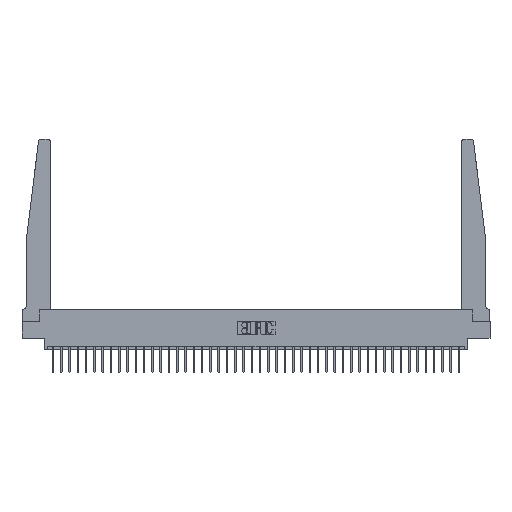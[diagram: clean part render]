
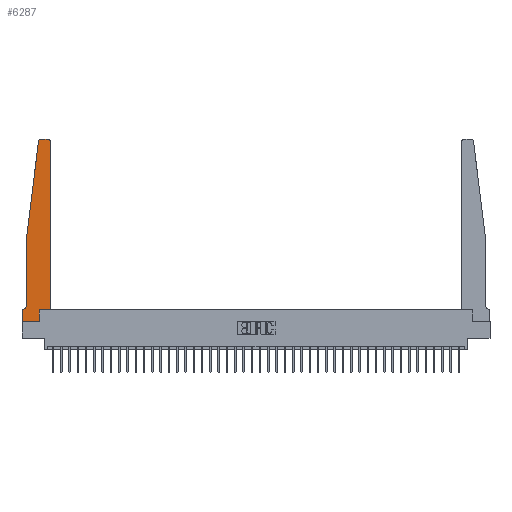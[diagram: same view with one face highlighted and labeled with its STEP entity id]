
A CAD part, top view. The second image highlights one B-rep face of the part: STEP entity #6287.
In plain terms, the highlighted planar face has unit normal (0, 0, 1).
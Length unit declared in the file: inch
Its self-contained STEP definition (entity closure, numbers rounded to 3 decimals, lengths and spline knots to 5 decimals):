
#651 = VECTOR ( 'NONE', #20652, 39.37008 ) ;
#763 = LINE ( 'NONE', #26192, #33918 ) ;
#776 = CARTESIAN_POINT ( 'NONE',  ( 0.27653, 2.75, 0.37 ) ) ;
#1004 = CARTESIAN_POINT ( 'NONE',  ( 0.065, 0.1875, 0.37 ) ) ;
#1012 = LINE ( 'NONE', #26637, #32268 ) ;
#1158 = VERTEX_POINT ( 'NONE', #13988 ) ;
#1454 = ORIENTED_EDGE ( 'NONE', *, *, #21829, .T. ) ;
#1738 = CIRCLE ( 'NONE', #35202, 0.03 ) ;
#1755 = EDGE_CURVE ( 'NONE', #35098, #30820, #1012, .T. ) ;
#3044 = CARTESIAN_POINT ( 'NONE',  ( 0.065, 0.2375, 0.37 ) ) ;
#3068 = ORIENTED_EDGE ( 'NONE', *, *, #21013, .T. ) ;
#3211 = CARTESIAN_POINT ( 'NONE',  ( 0.425, 0.18, 0.37 ) ) ;
#3277 = VERTEX_POINT ( 'NONE', #3044 ) ;
#4157 = DIRECTION ( 'NONE',  ( -1., 0., 0. ) ) ;
#4281 = LINE ( 'NONE', #32141, #19130 ) ;
#5537 = DIRECTION ( 'NONE',  ( 1., 0., 0. ) ) ;
#5551 = ORIENTED_EDGE ( 'NONE', *, *, #36770, .T. ) ;
#5706 = ORIENTED_EDGE ( 'NONE', *, *, #26764, .T. ) ;
#5817 = ORIENTED_EDGE ( 'NONE', *, *, #1755, .T. ) ;
#5936 = AXIS2_PLACEMENT_3D ( 'NONE', #36060, #19038, #24821 ) ;
#6287 = ADVANCED_FACE ( 'NONE', ( #8143 ), #28717, .T. ) ;
#6332 = VERTEX_POINT ( 'NONE', #16947 ) ;
#6560 = DIRECTION ( 'NONE',  ( 0., 1., 0. ) ) ;
#6620 = LINE ( 'NONE', #12411, #7082 ) ;
#7082 = VECTOR ( 'NONE', #14839, 39.37008 ) ;
#7101 = VECTOR ( 'NONE', #23597, 39.37008 ) ;
#7156 = VECTOR ( 'NONE', #35721, 39.37008 ) ;
#8001 = DIRECTION ( 'NONE',  ( 0., 0., 1. ) ) ;
#8143 = FACE_OUTER_BOUND ( 'NONE', #19870, .T. ) ;
#8250 = EDGE_CURVE ( 'NONE', #3277, #36630, #20712, .T. ) ;
#9331 = DIRECTION ( 'NONE',  ( 0., -1., 0. ) ) ;
#9425 = ORIENTED_EDGE ( 'NONE', *, *, #29002, .T. ) ;
#10098 = CIRCLE ( 'NONE', #5936, 0.03 ) ;
#10587 = CARTESIAN_POINT ( 'NONE',  ( 0.24675, 2.72367, 0.37 ) ) ;
#11297 = CARTESIAN_POINT ( 'NONE',  ( 0.425, 0.18, 0.37 ) ) ;
#11509 = CARTESIAN_POINT ( 'NONE',  ( 0., 0.1875, 0.37 ) ) ;
#11864 = VERTEX_POINT ( 'NONE', #14328 ) ;
#12101 = LINE ( 'NONE', #23685, #22616 ) ;
#12243 = DIRECTION ( 'NONE',  ( 1., 0., 0. ) ) ;
#12411 = CARTESIAN_POINT ( 'NONE',  ( 0.065, 1.25, 0.37 ) ) ;
#12468 = DIRECTION ( 'NONE',  ( -0.122, -0.992, 0. ) ) ;
#13988 = CARTESIAN_POINT ( 'NONE',  ( 0.425, 0.18, 0.37 ) ) ;
#14328 = CARTESIAN_POINT ( 'NONE',  ( 0.395, 2.75, 0.37 ) ) ;
#14839 = DIRECTION ( 'NONE',  ( 0., -1., 0. ) ) ;
#16272 = VERTEX_POINT ( 'NONE', #10587 ) ;
#16416 = DIRECTION ( 'NONE',  ( 1., 0., 0. ) ) ;
#16947 = CARTESIAN_POINT ( 'NONE',  ( 0.425, 2.72, 0.37 ) ) ;
#17515 = EDGE_CURVE ( 'NONE', #30820, #25981, #763, .T. ) ;
#18211 = ORIENTED_EDGE ( 'NONE', *, *, #29478, .T. ) ;
#18327 = ORIENTED_EDGE ( 'NONE', *, *, #20433, .T. ) ;
#19038 = DIRECTION ( 'NONE',  ( 0., 0., 1. ) ) ;
#19080 = CARTESIAN_POINT ( 'NONE',  ( 0.25, 2.75, 0.37 ) ) ;
#19130 = VECTOR ( 'NONE', #9331, 39.37008 ) ;
#19647 = VERTEX_POINT ( 'NONE', #24815 ) ;
#19728 = ORIENTED_EDGE ( 'NONE', *, *, #21038, .T. ) ;
#19870 = EDGE_LOOP ( 'NONE', ( #5551, #3068, #18211, #18327, #22497, #1454, #9425, #5817, #32576, #5706, #35235, #19728 ) ) ;
#20433 = EDGE_CURVE ( 'NONE', #34591, #3277, #6620, .T. ) ;
#20447 = DIRECTION ( 'NONE',  ( 0., 0., -1. ) ) ;
#20610 = LINE ( 'NONE', #3211, #7101 ) ;
#20652 = DIRECTION ( 'NONE',  ( -1., 0., 0. ) ) ;
#20712 = CIRCLE ( 'NONE', #23106, 0.05 ) ;
#21013 = EDGE_CURVE ( 'NONE', #36712, #16272, #10098, .T. ) ;
#21038 = EDGE_CURVE ( 'NONE', #6332, #11864, #1738, .T. ) ;
#21088 = CARTESIAN_POINT ( 'NONE',  ( 0.065, 1.25, 0.37 ) ) ;
#21829 = EDGE_CURVE ( 'NONE', #36630, #19647, #34870, .T. ) ;
#22497 = ORIENTED_EDGE ( 'NONE', *, *, #8250, .T. ) ;
#22616 = VECTOR ( 'NONE', #12468, 39.37008 ) ;
#23106 = AXIS2_PLACEMENT_3D ( 'NONE', #26609, #20447, #4157 ) ;
#23597 = DIRECTION ( 'NONE',  ( 0., 1., 0. ) ) ;
#23685 = CARTESIAN_POINT ( 'NONE',  ( 0.065, 1.25, 0.37 ) ) ;
#24309 = LINE ( 'NONE', #19080, #7156 ) ;
#24815 = CARTESIAN_POINT ( 'NONE',  ( 0., 0.1875, 0.37 ) ) ;
#24821 = DIRECTION ( 'NONE',  ( 1., 0., 0. ) ) ;
#25837 = CARTESIAN_POINT ( 'NONE',  ( 0.015, 0.1875, 0.37 ) ) ;
#25981 = VERTEX_POINT ( 'NONE', #34240 ) ;
#26192 = CARTESIAN_POINT ( 'NONE',  ( 0.2605, 0.18, 0.37 ) ) ;
#26436 = VECTOR ( 'NONE', #33202, 39.37008 ) ;
#26609 = CARTESIAN_POINT ( 'NONE',  ( 0.015, 0.2375, 0.37 ) ) ;
#26637 = CARTESIAN_POINT ( 'NONE',  ( 0., 0., 0.37 ) ) ;
#26764 = EDGE_CURVE ( 'NONE', #25981, #1158, #33934, .T. ) ;
#28169 = DIRECTION ( 'NONE',  ( 0., 0., 1. ) ) ;
#28436 = EDGE_CURVE ( 'NONE', #1158, #6332, #20610, .T. ) ;
#28717 = PLANE ( 'NONE',  #35727 ) ;
#29002 = EDGE_CURVE ( 'NONE', #19647, #35098, #4281, .T. ) ;
#29478 = EDGE_CURVE ( 'NONE', #16272, #34591, #12101, .T. ) ;
#30820 = VERTEX_POINT ( 'NONE', #35060 ) ;
#32033 = CARTESIAN_POINT ( 'NONE',  ( 0., 0., 0.37 ) ) ;
#32141 = CARTESIAN_POINT ( 'NONE',  ( 0., 0., 0.37 ) ) ;
#32268 = VECTOR ( 'NONE', #12243, 39.37008 ) ;
#32576 = ORIENTED_EDGE ( 'NONE', *, *, #17515, .T. ) ;
#33080 = CARTESIAN_POINT ( 'NONE',  ( 0.395, 2.72, 0.37 ) ) ;
#33202 = DIRECTION ( 'NONE',  ( 1., 0., 0. ) ) ;
#33918 = VECTOR ( 'NONE', #6560, 39.37008 ) ;
#33934 = LINE ( 'NONE', #11297, #26436 ) ;
#34240 = CARTESIAN_POINT ( 'NONE',  ( 0.2605, 0.18, 0.37 ) ) ;
#34591 = VERTEX_POINT ( 'NONE', #21088 ) ;
#34870 = LINE ( 'NONE', #1004, #651 ) ;
#35060 = CARTESIAN_POINT ( 'NONE',  ( 0.2605, 0., 0.37 ) ) ;
#35098 = VERTEX_POINT ( 'NONE', #32033 ) ;
#35202 = AXIS2_PLACEMENT_3D ( 'NONE', #33080, #8001, #16416 ) ;
#35235 = ORIENTED_EDGE ( 'NONE', *, *, #28436, .T. ) ;
#35721 = DIRECTION ( 'NONE',  ( -1., 0., 0. ) ) ;
#35727 = AXIS2_PLACEMENT_3D ( 'NONE', #11509, #28169, #5537 ) ;
#36060 = CARTESIAN_POINT ( 'NONE',  ( 0.27653, 2.72, 0.37 ) ) ;
#36630 = VERTEX_POINT ( 'NONE', #25837 ) ;
#36712 = VERTEX_POINT ( 'NONE', #776 ) ;
#36770 = EDGE_CURVE ( 'NONE', #11864, #36712, #24309, .T. ) ;
